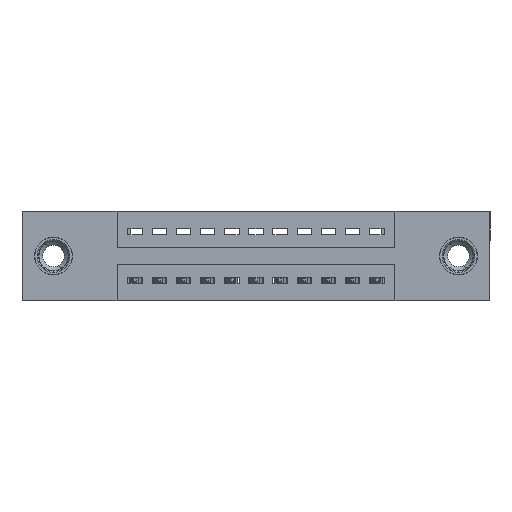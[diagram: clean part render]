
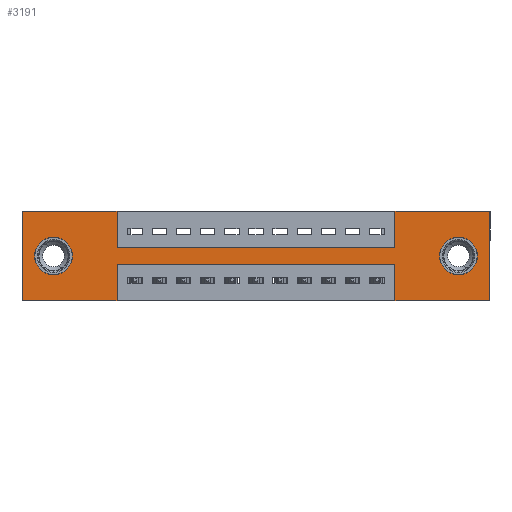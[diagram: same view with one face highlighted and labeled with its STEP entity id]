
A CAD part, front view. The second image highlights one B-rep face of the part: STEP entity #3191.
In plain terms, the highlighted planar face has unit normal (0, -1, 0).
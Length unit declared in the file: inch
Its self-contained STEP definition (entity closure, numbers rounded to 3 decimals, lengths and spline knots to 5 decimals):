
#48 = CARTESIAN_POINT ( 'NONE',  ( 0., 0., 0. ) ) ;
#346 = DIRECTION ( 'NONE',  ( -1., 0., 0. ) ) ;
#359 = EDGE_CURVE ( 'NONE', #893, #1582, #13092, .T. ) ;
#453 = CARTESIAN_POINT ( 'NONE',  ( 0., 0., -0.37 ) ) ;
#835 = VECTOR ( 'NONE', #3511, 39.37008 ) ;
#893 = VERTEX_POINT ( 'NONE', #5971 ) ;
#1006 = DIRECTION ( 'NONE',  ( 0., 0., -1. ) ) ;
#1204 = CARTESIAN_POINT ( 'NONE',  ( 0.3925, 0., -0.22 ) ) ;
#1315 = VECTOR ( 'NONE', #6516, 39.37008 ) ;
#1330 = CARTESIAN_POINT ( 'NONE',  ( 0.3925, 0., -0.15 ) ) ;
#1375 = EDGE_CURVE ( 'NONE', #12956, #6101, #1435, .T. ) ;
#1435 = LINE ( 'NONE', #13556, #14173 ) ;
#1505 = DIRECTION ( 'NONE',  ( 0., -1., 0. ) ) ;
#1552 = CARTESIAN_POINT ( 'NONE',  ( 1.5425, 0., 0. ) ) ;
#1582 = VERTEX_POINT ( 'NONE', #8014 ) ;
#1788 = DIRECTION ( 'NONE',  ( 0., 1., 0. ) ) ;
#2009 = CARTESIAN_POINT ( 'NONE',  ( 1.805, 0., -0.185 ) ) ;
#2018 = CARTESIAN_POINT ( 'NONE',  ( 1.5425, 0., 0. ) ) ;
#2194 = DIRECTION ( 'NONE',  ( -1., 0., 0. ) ) ;
#2212 = DIRECTION ( 'NONE',  ( -1., 0., 0. ) ) ;
#2376 = EDGE_CURVE ( 'NONE', #5642, #13305, #4072, .T. ) ;
#2438 = DIRECTION ( 'NONE',  ( 1., 0., 0. ) ) ;
#2458 = ORIENTED_EDGE ( 'NONE', *, *, #6323, .F. ) ;
#2462 = LINE ( 'NONE', #13285, #14115 ) ;
#2554 = LINE ( 'NONE', #8245, #6457 ) ;
#2715 = DIRECTION ( 'NONE',  ( 0., 1., 0. ) ) ;
#2862 = CARTESIAN_POINT ( 'NONE',  ( 1.935, 0., 0. ) ) ;
#2876 = EDGE_CURVE ( 'NONE', #12813, #6913, #7590, .T. ) ;
#3091 = ORIENTED_EDGE ( 'NONE', *, *, #12933, .F. ) ;
#3171 = VERTEX_POINT ( 'NONE', #10018 ) ;
#3191 = ADVANCED_FACE ( 'NONE', ( #13958, #14123, #7928 ), #10587, .T. ) ;
#3406 = VERTEX_POINT ( 'NONE', #4643 ) ;
#3511 = DIRECTION ( 'NONE',  ( 1., 0., 0. ) ) ;
#3714 = LINE ( 'NONE', #2862, #12230 ) ;
#4000 = ORIENTED_EDGE ( 'NONE', *, *, #8097, .F. ) ;
#4039 = LINE ( 'NONE', #48, #835 ) ;
#4047 = EDGE_LOOP ( 'NONE', ( #6914, #9802 ) ) ;
#4072 = CIRCLE ( 'NONE', #10127, 0.078 ) ;
#4219 = DIRECTION ( 'NONE',  ( 0., 0., -1. ) ) ;
#4354 = CARTESIAN_POINT ( 'NONE',  ( 1.5425, 0., -0.37 ) ) ;
#4424 = CARTESIAN_POINT ( 'NONE',  ( 0.3925, 0., -0.37 ) ) ;
#4517 = CARTESIAN_POINT ( 'NONE',  ( 0., 0., 0. ) ) ;
#4546 = VECTOR ( 'NONE', #5405, 39.37008 ) ;
#4620 = ORIENTED_EDGE ( 'NONE', *, *, #5426, .F. ) ;
#4643 = CARTESIAN_POINT ( 'NONE',  ( 0.3925, 0., -0.37 ) ) ;
#5396 = CARTESIAN_POINT ( 'NONE',  ( 0., 0., 0. ) ) ;
#5405 = DIRECTION ( 'NONE',  ( 0., 0., 1. ) ) ;
#5426 = EDGE_CURVE ( 'NONE', #6101, #6735, #6650, .T. ) ;
#5456 = VERTEX_POINT ( 'NONE', #6670 ) ;
#5546 = CARTESIAN_POINT ( 'NONE',  ( 0., 0., -0.37 ) ) ;
#5642 = VERTEX_POINT ( 'NONE', #9062 ) ;
#5952 = CARTESIAN_POINT ( 'NONE',  ( 0.13, 0., -0.263 ) ) ;
#5971 = CARTESIAN_POINT ( 'NONE',  ( 0.3925, 0., -0.15 ) ) ;
#6061 = ORIENTED_EDGE ( 'NONE', *, *, #14084, .F. ) ;
#6101 = VERTEX_POINT ( 'NONE', #4354 ) ;
#6133 = ORIENTED_EDGE ( 'NONE', *, *, #12209, .F. ) ;
#6228 = CARTESIAN_POINT ( 'NONE',  ( 1.5425, 0., -0.22 ) ) ;
#6323 = EDGE_CURVE ( 'NONE', #6735, #13846, #2554, .T. ) ;
#6374 = DIRECTION ( 'NONE',  ( 0., 0., 1. ) ) ;
#6457 = VECTOR ( 'NONE', #346, 39.37008 ) ;
#6506 = DIRECTION ( 'NONE',  ( 0., 1., 0. ) ) ;
#6516 = DIRECTION ( 'NONE',  ( 0., 0., 1. ) ) ;
#6628 = AXIS2_PLACEMENT_3D ( 'NONE', #9557, #1788, #14238 ) ;
#6650 = LINE ( 'NONE', #12251, #1315 ) ;
#6670 = CARTESIAN_POINT ( 'NONE',  ( 0., 0., -0.37 ) ) ;
#6680 = DIRECTION ( 'NONE',  ( 0., 0., -1. ) ) ;
#6735 = VERTEX_POINT ( 'NONE', #6228 ) ;
#6803 = ORIENTED_EDGE ( 'NONE', *, *, #10900, .F. ) ;
#6896 = CARTESIAN_POINT ( 'NONE',  ( 1.935, 0., -0.37 ) ) ;
#6913 = VERTEX_POINT ( 'NONE', #14278 ) ;
#6914 = ORIENTED_EDGE ( 'NONE', *, *, #2376, .T. ) ;
#7035 = ORIENTED_EDGE ( 'NONE', *, *, #2876, .T. ) ;
#7050 = DIRECTION ( 'NONE',  ( 0., 0., -1. ) ) ;
#7081 = EDGE_CURVE ( 'NONE', #13305, #5642, #12790, .T. ) ;
#7154 = VERTEX_POINT ( 'NONE', #4517 ) ;
#7338 = EDGE_CURVE ( 'NONE', #3406, #5456, #13252, .T. ) ;
#7590 = CIRCLE ( 'NONE', #10399, 0.078 ) ;
#7807 = EDGE_CURVE ( 'NONE', #9569, #893, #2462, .T. ) ;
#7928 = FACE_OUTER_BOUND ( 'NONE', #10756, .T. ) ;
#8014 = CARTESIAN_POINT ( 'NONE',  ( 1.5425, 0., -0.15 ) ) ;
#8097 = EDGE_CURVE ( 'NONE', #1582, #8173, #13569, .T. ) ;
#8173 = VERTEX_POINT ( 'NONE', #1552 ) ;
#8245 = CARTESIAN_POINT ( 'NONE',  ( 0.3925, 0., -0.22 ) ) ;
#8312 = VECTOR ( 'NONE', #2438, 39.37008 ) ;
#8657 = ORIENTED_EDGE ( 'NONE', *, *, #9117, .T. ) ;
#9062 = CARTESIAN_POINT ( 'NONE',  ( 1.805, 0., -0.107 ) ) ;
#9117 = EDGE_CURVE ( 'NONE', #6913, #12813, #11416, .T. ) ;
#9557 = CARTESIAN_POINT ( 'NONE',  ( 0.13, 0., -0.185 ) ) ;
#9569 = VERTEX_POINT ( 'NONE', #10736 ) ;
#9802 = ORIENTED_EDGE ( 'NONE', *, *, #7081, .T. ) ;
#9853 = ORIENTED_EDGE ( 'NONE', *, *, #10728, .F. ) ;
#9975 = AXIS2_PLACEMENT_3D ( 'NONE', #453, #1505, #7050 ) ;
#9981 = CARTESIAN_POINT ( 'NONE',  ( 1.805, 0., -0.185 ) ) ;
#10018 = CARTESIAN_POINT ( 'NONE',  ( 1.935, 0., 0. ) ) ;
#10127 = AXIS2_PLACEMENT_3D ( 'NONE', #2009, #6506, #14353 ) ;
#10286 = CARTESIAN_POINT ( 'NONE',  ( 1.805, 0., -0.263 ) ) ;
#10399 = AXIS2_PLACEMENT_3D ( 'NONE', #14176, #2715, #14023 ) ;
#10587 = PLANE ( 'NONE',  #9975 ) ;
#10728 = EDGE_CURVE ( 'NONE', #5456, #7154, #14027, .T. ) ;
#10736 = CARTESIAN_POINT ( 'NONE',  ( 0.3925, 0., 0. ) ) ;
#10756 = EDGE_LOOP ( 'NONE', ( #3091, #2458, #4620, #13301, #6133, #6061, #4000, #11950, #13426, #6803, #9853, #12048 ) ) ;
#10900 = EDGE_CURVE ( 'NONE', #7154, #9569, #13134, .T. ) ;
#10930 = DIRECTION ( 'NONE',  ( 1., 0., 0. ) ) ;
#11143 = VECTOR ( 'NONE', #11224, 39.37008 ) ;
#11224 = DIRECTION ( 'NONE',  ( 0., 0., -1. ) ) ;
#11306 = AXIS2_PLACEMENT_3D ( 'NONE', #9981, #12310, #1006 ) ;
#11416 = CIRCLE ( 'NONE', #6628, 0.078 ) ;
#11950 = ORIENTED_EDGE ( 'NONE', *, *, #359, .F. ) ;
#12048 = ORIENTED_EDGE ( 'NONE', *, *, #7338, .F. ) ;
#12209 = EDGE_CURVE ( 'NONE', #3171, #12956, #3714, .T. ) ;
#12230 = VECTOR ( 'NONE', #4219, 39.37008 ) ;
#12234 = LINE ( 'NONE', #4424, #11143 ) ;
#12251 = CARTESIAN_POINT ( 'NONE',  ( 1.5425, 0., -0.37 ) ) ;
#12310 = DIRECTION ( 'NONE',  ( 0., 1., 0. ) ) ;
#12534 = EDGE_LOOP ( 'NONE', ( #8657, #7035 ) ) ;
#12790 = CIRCLE ( 'NONE', #11306, 0.078 ) ;
#12813 = VERTEX_POINT ( 'NONE', #5952 ) ;
#12907 = VECTOR ( 'NONE', #2194, 39.37008 ) ;
#12933 = EDGE_CURVE ( 'NONE', #13846, #3406, #12234, .T. ) ;
#12956 = VERTEX_POINT ( 'NONE', #6896 ) ;
#12966 = VECTOR ( 'NONE', #10930, 39.37008 ) ;
#13092 = LINE ( 'NONE', #1330, #8312 ) ;
#13134 = LINE ( 'NONE', #13513, #12966 ) ;
#13252 = LINE ( 'NONE', #5546, #12907 ) ;
#13285 = CARTESIAN_POINT ( 'NONE',  ( 0.3925, 0., 0. ) ) ;
#13301 = ORIENTED_EDGE ( 'NONE', *, *, #1375, .F. ) ;
#13305 = VERTEX_POINT ( 'NONE', #10286 ) ;
#13426 = ORIENTED_EDGE ( 'NONE', *, *, #7807, .F. ) ;
#13513 = CARTESIAN_POINT ( 'NONE',  ( 0., 0., 0. ) ) ;
#13556 = CARTESIAN_POINT ( 'NONE',  ( 0., 0., -0.37 ) ) ;
#13569 = LINE ( 'NONE', #2018, #4546 ) ;
#13846 = VERTEX_POINT ( 'NONE', #1204 ) ;
#13958 = FACE_BOUND ( 'NONE', #4047, .T. ) ;
#14023 = DIRECTION ( 'NONE',  ( 0., 0., 1. ) ) ;
#14027 = LINE ( 'NONE', #5396, #14553 ) ;
#14084 = EDGE_CURVE ( 'NONE', #8173, #3171, #4039, .T. ) ;
#14115 = VECTOR ( 'NONE', #6680, 39.37008 ) ;
#14123 = FACE_BOUND ( 'NONE', #12534, .T. ) ;
#14173 = VECTOR ( 'NONE', #2212, 39.37008 ) ;
#14176 = CARTESIAN_POINT ( 'NONE',  ( 0.13, 0., -0.185 ) ) ;
#14238 = DIRECTION ( 'NONE',  ( 0., 0., 1. ) ) ;
#14278 = CARTESIAN_POINT ( 'NONE',  ( 0.13, 0., -0.107 ) ) ;
#14353 = DIRECTION ( 'NONE',  ( 0., 0., -1. ) ) ;
#14553 = VECTOR ( 'NONE', #6374, 39.37008 ) ;
